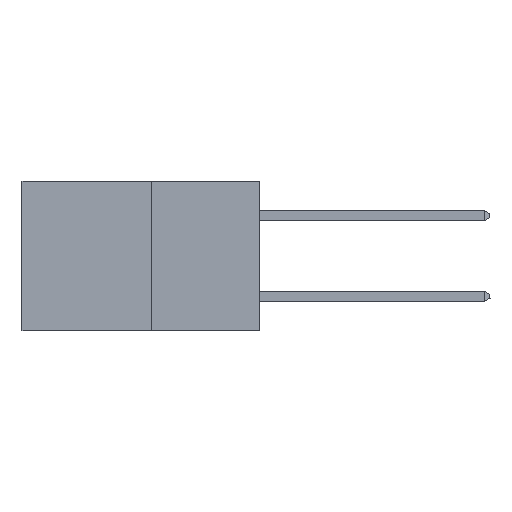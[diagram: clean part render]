
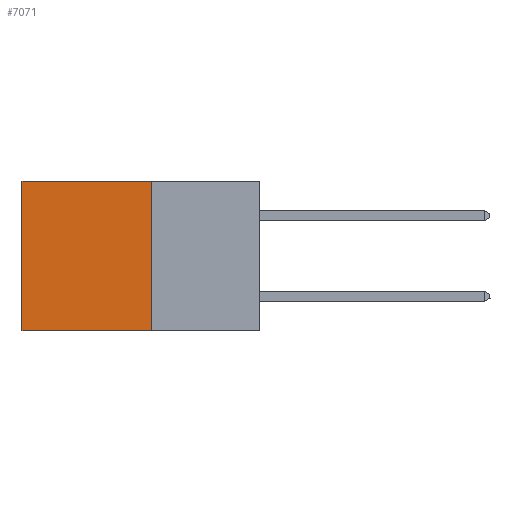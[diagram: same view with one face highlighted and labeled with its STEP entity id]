
A CAD part, left-side view. The second image highlights one B-rep face of the part: STEP entity #7071.
In plain terms, the highlighted planar face has unit normal (-1, 0, 0).
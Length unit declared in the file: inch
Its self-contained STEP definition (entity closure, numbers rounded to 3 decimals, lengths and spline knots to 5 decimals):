
#347 = VERTEX_POINT ( 'NONE', #11762 ) ;
#581 = CARTESIAN_POINT ( 'NONE',  ( 0.277, 0.27, -0.37 ) ) ;
#809 = VECTOR ( 'NONE', #6772, 39.37008 ) ;
#877 = VERTEX_POINT ( 'NONE', #15887 ) ;
#1141 = ORIENTED_EDGE ( 'NONE', *, *, #10915, .F. ) ;
#2018 = EDGE_LOOP ( 'NONE', ( #14383, #1141, #7404, #14329 ) ) ;
#2939 = PLANE ( 'NONE',  #11497 ) ;
#3461 = VERTEX_POINT ( 'NONE', #5550 ) ;
#5443 = DIRECTION ( 'NONE',  ( 0., 0., -1. ) ) ;
#5550 = CARTESIAN_POINT ( 'NONE',  ( 0.277, 0.59, -0.37 ) ) ;
#5986 = VECTOR ( 'NONE', #8097, 39.37008 ) ;
#6390 = LINE ( 'NONE', #581, #5986 ) ;
#6772 = DIRECTION ( 'NONE',  ( 0., 1., 0. ) ) ;
#7071 = ADVANCED_FACE ( 'NONE', ( #9847 ), #2939, .F. ) ;
#7101 = EDGE_CURVE ( 'NONE', #347, #3461, #9445, .T. ) ;
#7404 = ORIENTED_EDGE ( 'NONE', *, *, #16215, .F. ) ;
#7417 = CARTESIAN_POINT ( 'NONE',  ( 0.277, 0.27, -0.37 ) ) ;
#7982 = DIRECTION ( 'NONE',  ( 0., 0., -1. ) ) ;
#8097 = DIRECTION ( 'NONE',  ( 0., 0., -1. ) ) ;
#8227 = VERTEX_POINT ( 'NONE', #7417 ) ;
#9272 = CARTESIAN_POINT ( 'NONE',  ( 0.277, 0.59, -0.37 ) ) ;
#9445 = LINE ( 'NONE', #9272, #15723 ) ;
#9847 = FACE_OUTER_BOUND ( 'NONE', #2018, .T. ) ;
#10107 = VECTOR ( 'NONE', #11254, 39.37008 ) ;
#10459 = LINE ( 'NONE', #15563, #809 ) ;
#10915 = EDGE_CURVE ( 'NONE', #8227, #3461, #13072, .T. ) ;
#11254 = DIRECTION ( 'NONE',  ( 0., 1., 0. ) ) ;
#11497 = AXIS2_PLACEMENT_3D ( 'NONE', #11750, #12998, #5443 ) ;
#11750 = CARTESIAN_POINT ( 'NONE',  ( 0.277, 0.27, -0.37 ) ) ;
#11762 = CARTESIAN_POINT ( 'NONE',  ( 0.277, 0.59, 0. ) ) ;
#12257 = EDGE_CURVE ( 'NONE', #877, #347, #10459, .T. ) ;
#12514 = CARTESIAN_POINT ( 'NONE',  ( 0.277, 0.27, -0.37 ) ) ;
#12998 = DIRECTION ( 'NONE',  ( 1., 0., 0. ) ) ;
#13072 = LINE ( 'NONE', #12514, #10107 ) ;
#14329 = ORIENTED_EDGE ( 'NONE', *, *, #12257, .T. ) ;
#14383 = ORIENTED_EDGE ( 'NONE', *, *, #7101, .T. ) ;
#15563 = CARTESIAN_POINT ( 'NONE',  ( 0.277, 0.27, 0. ) ) ;
#15723 = VECTOR ( 'NONE', #7982, 39.37008 ) ;
#15887 = CARTESIAN_POINT ( 'NONE',  ( 0.277, 0.27, 0. ) ) ;
#16215 = EDGE_CURVE ( 'NONE', #877, #8227, #6390, .T. ) ;
